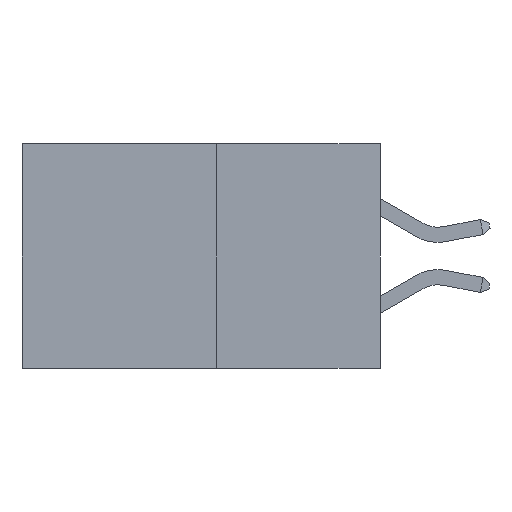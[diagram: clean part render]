
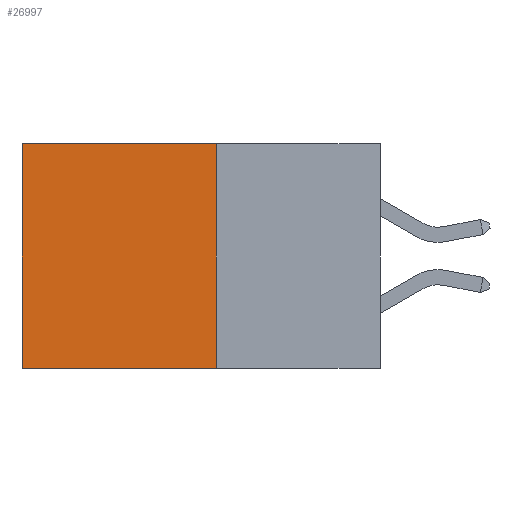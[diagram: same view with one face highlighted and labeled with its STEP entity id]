
A CAD part, left-side view. The second image highlights one B-rep face of the part: STEP entity #26997.
In plain terms, the highlighted planar face has unit normal (-1, 0, 0).
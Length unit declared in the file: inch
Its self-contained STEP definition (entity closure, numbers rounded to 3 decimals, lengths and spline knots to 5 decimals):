
#434 = VECTOR ( 'NONE', #10566, 39.37008 ) ;
#1624 = VECTOR ( 'NONE', #14982, 39.37008 ) ;
#1738 = CARTESIAN_POINT ( 'NONE',  ( 0.277, 0.27, -0.37 ) ) ;
#2021 = VECTOR ( 'NONE', #13231, 39.37008 ) ;
#2154 = EDGE_CURVE ( 'NONE', #26835, #7433, #10995, .T. ) ;
#3201 = VERTEX_POINT ( 'NONE', #18028 ) ;
#4299 = DIRECTION ( 'NONE',  ( 1., 0., 0. ) ) ;
#5487 = CARTESIAN_POINT ( 'NONE',  ( 0.277, 0.59, -0.37 ) ) ;
#6441 = AXIS2_PLACEMENT_3D ( 'NONE', #1738, #4299, #21940 ) ;
#7433 = VERTEX_POINT ( 'NONE', #9972 ) ;
#7456 = CARTESIAN_POINT ( 'NONE',  ( 0.277, 0.59, -0.37 ) ) ;
#8066 = ORIENTED_EDGE ( 'NONE', *, *, #18015, .T. ) ;
#8246 = CARTESIAN_POINT ( 'NONE',  ( 0.277, 0.27, 0. ) ) ;
#9972 = CARTESIAN_POINT ( 'NONE',  ( 0.277, 0.27, -0.37 ) ) ;
#10566 = DIRECTION ( 'NONE',  ( 0., 0., -1. ) ) ;
#10995 = LINE ( 'NONE', #24890, #30145 ) ;
#11434 = EDGE_CURVE ( 'NONE', #7433, #13420, #22167, .T. ) ;
#11668 = EDGE_CURVE ( 'NONE', #26835, #3201, #28360, .T. ) ;
#11797 = EDGE_LOOP ( 'NONE', ( #8066, #13710, #12558, #27579 ) ) ;
#12558 = ORIENTED_EDGE ( 'NONE', *, *, #2154, .F. ) ;
#12646 = FACE_OUTER_BOUND ( 'NONE', #11797, .T. ) ;
#13051 = LINE ( 'NONE', #5487, #434 ) ;
#13231 = DIRECTION ( 'NONE',  ( 0., 1., 0. ) ) ;
#13304 = CARTESIAN_POINT ( 'NONE',  ( 0.277, 0.27, -0.37 ) ) ;
#13420 = VERTEX_POINT ( 'NONE', #7456 ) ;
#13710 = ORIENTED_EDGE ( 'NONE', *, *, #11434, .F. ) ;
#14753 = CARTESIAN_POINT ( 'NONE',  ( 0.277, 0.27, 0. ) ) ;
#14982 = DIRECTION ( 'NONE',  ( 0., 1., 0. ) ) ;
#18015 = EDGE_CURVE ( 'NONE', #3201, #13420, #13051, .T. ) ;
#18028 = CARTESIAN_POINT ( 'NONE',  ( 0.277, 0.59, 0. ) ) ;
#19412 = PLANE ( 'NONE',  #6441 ) ;
#21657 = DIRECTION ( 'NONE',  ( 0., 0., -1. ) ) ;
#21940 = DIRECTION ( 'NONE',  ( 0., 0., -1. ) ) ;
#22167 = LINE ( 'NONE', #13304, #2021 ) ;
#24890 = CARTESIAN_POINT ( 'NONE',  ( 0.277, 0.27, -0.37 ) ) ;
#26835 = VERTEX_POINT ( 'NONE', #8246 ) ;
#26997 = ADVANCED_FACE ( 'NONE', ( #12646 ), #19412, .F. ) ;
#27579 = ORIENTED_EDGE ( 'NONE', *, *, #11668, .T. ) ;
#28360 = LINE ( 'NONE', #14753, #1624 ) ;
#30145 = VECTOR ( 'NONE', #21657, 39.37008 ) ;
